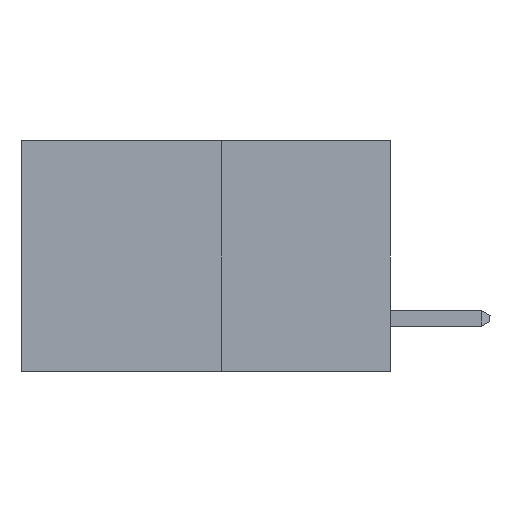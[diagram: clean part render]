
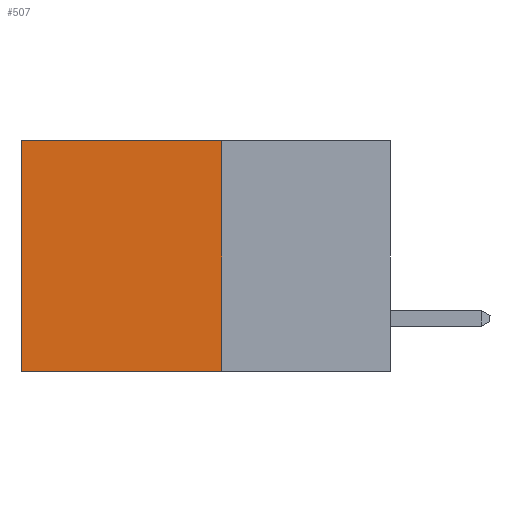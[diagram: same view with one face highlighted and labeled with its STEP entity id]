
A CAD part, left-side view. The second image highlights one B-rep face of the part: STEP entity #507.
In plain terms, the highlighted planar face has unit normal (-1, 0, 0).
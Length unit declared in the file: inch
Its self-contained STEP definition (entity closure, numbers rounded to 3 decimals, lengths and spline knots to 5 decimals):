
#507 = ADVANCED_FACE ( 'NONE', ( #8641 ), #11061, .F. ) ;
#1279 = EDGE_CURVE ( 'NONE', #2706, #7947, #4902, .T. ) ;
#1592 = VECTOR ( 'NONE', #9755, 39.37008 ) ;
#1786 = EDGE_CURVE ( 'NONE', #4445, #2656, #8879, .T. ) ;
#1931 = CARTESIAN_POINT ( 'NONE',  ( 0.277, 0.27, -0.37 ) ) ;
#2656 = VERTEX_POINT ( 'NONE', #8596 ) ;
#2706 = VERTEX_POINT ( 'NONE', #8511 ) ;
#3311 = CARTESIAN_POINT ( 'NONE',  ( 0.277, 0.27, -0.37 ) ) ;
#4445 = VERTEX_POINT ( 'NONE', #1931 ) ;
#4902 = LINE ( 'NONE', #11218, #6122 ) ;
#5182 = CARTESIAN_POINT ( 'NONE',  ( 0.277, 0.59, -0.37 ) ) ;
#5684 = EDGE_LOOP ( 'NONE', ( #6484, #7163, #7847, #9874 ) ) ;
#5734 = DIRECTION ( 'NONE',  ( 0., 1., 0. ) ) ;
#5994 = DIRECTION ( 'NONE',  ( 1., 0., 0. ) ) ;
#6009 = DIRECTION ( 'NONE',  ( 0., 0., -1. ) ) ;
#6122 = VECTOR ( 'NONE', #5734, 39.37008 ) ;
#6373 = CARTESIAN_POINT ( 'NONE',  ( 0.277, 0.59, 0. ) ) ;
#6484 = ORIENTED_EDGE ( 'NONE', *, *, #8167, .T. ) ;
#6731 = VECTOR ( 'NONE', #8625, 39.37008 ) ;
#7163 = ORIENTED_EDGE ( 'NONE', *, *, #1786, .F. ) ;
#7271 = CARTESIAN_POINT ( 'NONE',  ( 0.277, 0.27, -0.37 ) ) ;
#7300 = LINE ( 'NONE', #5182, #9421 ) ;
#7847 = ORIENTED_EDGE ( 'NONE', *, *, #10086, .F. ) ;
#7947 = VERTEX_POINT ( 'NONE', #6373 ) ;
#8167 = EDGE_CURVE ( 'NONE', #7947, #2656, #7300, .T. ) ;
#8339 = AXIS2_PLACEMENT_3D ( 'NONE', #11748, #5994, #6009 ) ;
#8511 = CARTESIAN_POINT ( 'NONE',  ( 0.277, 0.27, 0. ) ) ;
#8596 = CARTESIAN_POINT ( 'NONE',  ( 0.277, 0.59, -0.37 ) ) ;
#8625 = DIRECTION ( 'NONE',  ( 0., 0., -1. ) ) ;
#8641 = FACE_OUTER_BOUND ( 'NONE', #5684, .T. ) ;
#8879 = LINE ( 'NONE', #7271, #1592 ) ;
#9112 = LINE ( 'NONE', #3311, #6731 ) ;
#9421 = VECTOR ( 'NONE', #9593, 39.37008 ) ;
#9593 = DIRECTION ( 'NONE',  ( 0., 0., -1. ) ) ;
#9755 = DIRECTION ( 'NONE',  ( 0., 1., 0. ) ) ;
#9874 = ORIENTED_EDGE ( 'NONE', *, *, #1279, .T. ) ;
#10086 = EDGE_CURVE ( 'NONE', #2706, #4445, #9112, .T. ) ;
#11061 = PLANE ( 'NONE',  #8339 ) ;
#11218 = CARTESIAN_POINT ( 'NONE',  ( 0.277, 0.27, 0. ) ) ;
#11748 = CARTESIAN_POINT ( 'NONE',  ( 0.277, 0.27, -0.37 ) ) ;
